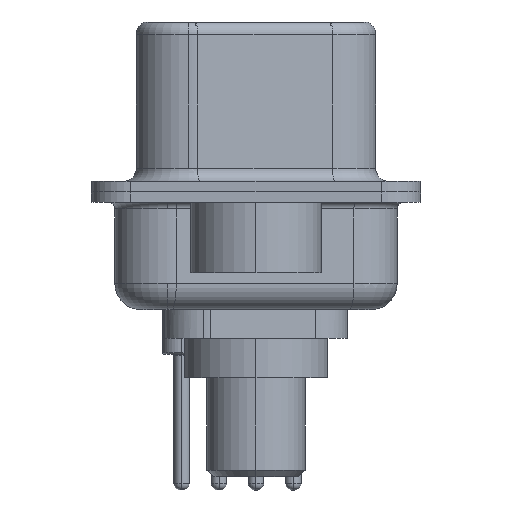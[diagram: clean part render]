
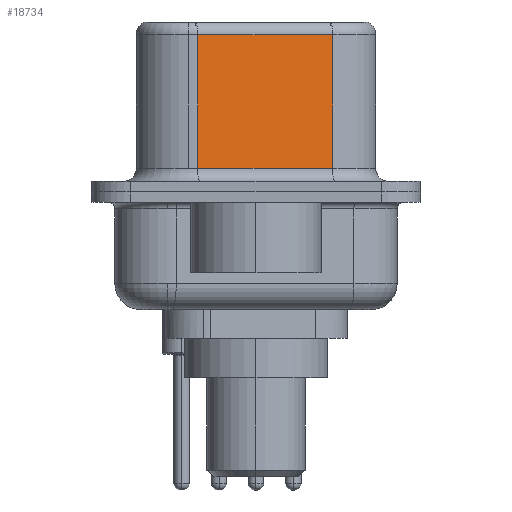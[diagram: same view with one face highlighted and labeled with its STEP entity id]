
A CAD part, left-side view. The second image highlights one B-rep face of the part: STEP entity #18734.
In plain terms, the highlighted planar face has unit normal (-0.985, -0.174, 0).
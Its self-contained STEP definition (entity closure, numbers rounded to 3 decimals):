
#246 = EDGE_CURVE ( 'NONE', #15392, #6512, #6028, .T. ) ;
#274 = VECTOR ( 'NONE', #19835, 1000. ) ;
#878 = EDGE_LOOP ( 'NONE', ( #1045, #15903, #8859, #11836 ) ) ;
#1045 = ORIENTED_EDGE ( 'NONE', *, *, #246, .F. ) ;
#1293 = VECTOR ( 'NONE', #8264, 1000. ) ;
#1340 = EDGE_CURVE ( 'NONE', #12758, #6512, #14436, .T. ) ;
#2815 = VERTEX_POINT ( 'NONE', #6886 ) ;
#2925 = CARTESIAN_POINT ( 'NONE',  ( 4.58, -2.927, 6.02 ) ) ;
#4170 = LINE ( 'NONE', #17966, #16615 ) ;
#5534 = LINE ( 'NONE', #9736, #1293 ) ;
#6028 = LINE ( 'NONE', #11905, #274 ) ;
#6512 = VERTEX_POINT ( 'NONE', #12504 ) ;
#6886 = CARTESIAN_POINT ( 'NONE',  ( 3.67, 2.233, 6.02 ) ) ;
#8264 = DIRECTION ( 'NONE',  ( -0.174, 0.985, 0. ) ) ;
#8649 = DIRECTION ( 'NONE',  ( 0., 0., -1. ) ) ;
#8859 = ORIENTED_EDGE ( 'NONE', *, *, #19134, .T. ) ;
#8876 = CARTESIAN_POINT ( 'NONE',  ( 3.67, 2.233, 0.9 ) ) ;
#9335 = CARTESIAN_POINT ( 'NONE',  ( 4.58, -2.927, 6.52 ) ) ;
#9736 = CARTESIAN_POINT ( 'NONE',  ( 4.58, -2.927, 6.02 ) ) ;
#9829 = EDGE_CURVE ( 'NONE', #15392, #2815, #5534, .T. ) ;
#10879 = PLANE ( 'NONE',  #17458 ) ;
#11836 = ORIENTED_EDGE ( 'NONE', *, *, #1340, .T. ) ;
#11905 = CARTESIAN_POINT ( 'NONE',  ( 4.58, -2.927, 6.52 ) ) ;
#12452 = DIRECTION ( 'NONE',  ( -0.174, 0.985, 0. ) ) ;
#12504 = CARTESIAN_POINT ( 'NONE',  ( 4.58, -2.927, 0.9 ) ) ;
#12758 = VERTEX_POINT ( 'NONE', #8876 ) ;
#14436 = LINE ( 'NONE', #15667, #18106 ) ;
#15392 = VERTEX_POINT ( 'NONE', #2925 ) ;
#15491 = DIRECTION ( 'NONE',  ( 0.985, 0.174, 0. ) ) ;
#15667 = CARTESIAN_POINT ( 'NONE',  ( 4.58, -2.927, 0.9 ) ) ;
#15903 = ORIENTED_EDGE ( 'NONE', *, *, #9829, .T. ) ;
#16514 = DIRECTION ( 'NONE',  ( 0.174, -0.985, 0. ) ) ;
#16615 = VECTOR ( 'NONE', #8649, 1000. ) ;
#17374 = FACE_OUTER_BOUND ( 'NONE', #878, .T. ) ;
#17458 = AXIS2_PLACEMENT_3D ( 'NONE', #9335, #15491, #12452 ) ;
#17966 = CARTESIAN_POINT ( 'NONE',  ( 3.67, 2.233, 6.52 ) ) ;
#18106 = VECTOR ( 'NONE', #16514, 1000. ) ;
#18734 = ADVANCED_FACE ( 'NONE', ( #17374 ), #10879, .F. ) ;
#19134 = EDGE_CURVE ( 'NONE', #2815, #12758, #4170, .T. ) ;
#19835 = DIRECTION ( 'NONE',  ( 0., 0., -1. ) ) ;
